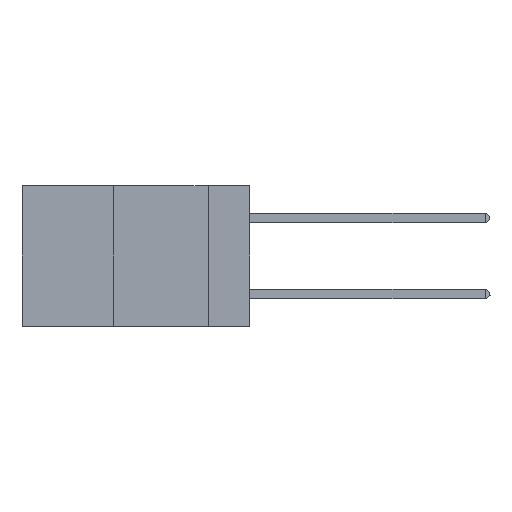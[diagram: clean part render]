
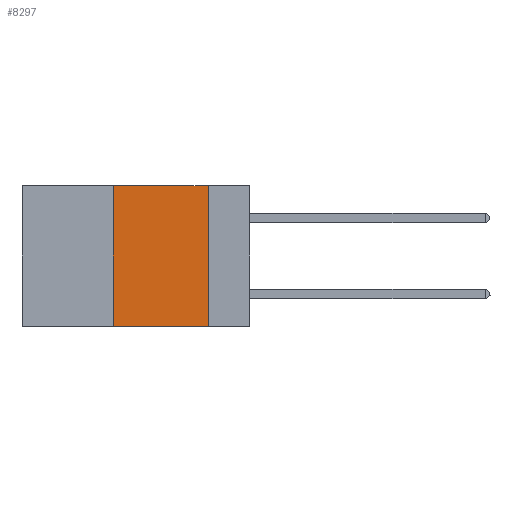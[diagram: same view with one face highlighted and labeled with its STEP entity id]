
A CAD part, left-side view. The second image highlights one B-rep face of the part: STEP entity #8297.
In plain terms, the highlighted planar face has unit normal (-1, 0, 0).
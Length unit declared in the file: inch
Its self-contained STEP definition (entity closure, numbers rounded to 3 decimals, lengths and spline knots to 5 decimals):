
#492 = DIRECTION ( 'NONE',  ( 0., 0., 1. ) ) ;
#702 = VECTOR ( 'NONE', #6221, 39.37008 ) ;
#776 = ORIENTED_EDGE ( 'NONE', *, *, #14512, .F. ) ;
#954 = EDGE_LOOP ( 'NONE', ( #1184, #1375, #776, #11530 ) ) ;
#1025 = CARTESIAN_POINT ( 'NONE',  ( 0., 0.11, 0. ) ) ;
#1184 = ORIENTED_EDGE ( 'NONE', *, *, #7351, .F. ) ;
#1375 = ORIENTED_EDGE ( 'NONE', *, *, #3926, .F. ) ;
#1464 = CARTESIAN_POINT ( 'NONE',  ( 0., 0.11, -0.37 ) ) ;
#1630 = CARTESIAN_POINT ( 'NONE',  ( 0., 0.36, 0. ) ) ;
#2673 = VECTOR ( 'NONE', #4541, 39.37008 ) ;
#2970 = VERTEX_POINT ( 'NONE', #3033 ) ;
#3033 = CARTESIAN_POINT ( 'NONE',  ( 0., 0.36, -0.37 ) ) ;
#3047 = CARTESIAN_POINT ( 'NONE',  ( 0., 0.6, 0. ) ) ;
#3343 = CARTESIAN_POINT ( 'NONE',  ( 0., 0.11, 0. ) ) ;
#3744 = VERTEX_POINT ( 'NONE', #1464 ) ;
#3909 = CARTESIAN_POINT ( 'NONE',  ( 0., 0.6, -0.37 ) ) ;
#3926 = EDGE_CURVE ( 'NONE', #8511, #8429, #7012, .T. ) ;
#4541 = DIRECTION ( 'NONE',  ( 0., 0., -1. ) ) ;
#6221 = DIRECTION ( 'NONE',  ( 0., -1., 0. ) ) ;
#6929 = CARTESIAN_POINT ( 'NONE',  ( 0., 0.36, 0. ) ) ;
#7012 = LINE ( 'NONE', #15236, #8849 ) ;
#7351 = EDGE_CURVE ( 'NONE', #8429, #3744, #13919, .T. ) ;
#7542 = LINE ( 'NONE', #1630, #14424 ) ;
#8297 = ADVANCED_FACE ( 'NONE', ( #9582 ), #10255, .F. ) ;
#8429 = VERTEX_POINT ( 'NONE', #1025 ) ;
#8511 = VERTEX_POINT ( 'NONE', #6929 ) ;
#8849 = VECTOR ( 'NONE', #14131, 39.37008 ) ;
#9582 = FACE_OUTER_BOUND ( 'NONE', #954, .T. ) ;
#9937 = LINE ( 'NONE', #3909, #702 ) ;
#10255 = PLANE ( 'NONE',  #12591 ) ;
#11530 = ORIENTED_EDGE ( 'NONE', *, *, #14895, .T. ) ;
#12591 = AXIS2_PLACEMENT_3D ( 'NONE', #3047, #13897, #15010 ) ;
#13897 = DIRECTION ( 'NONE',  ( 1., 0., 0. ) ) ;
#13919 = LINE ( 'NONE', #3343, #2673 ) ;
#14131 = DIRECTION ( 'NONE',  ( 0., -1., 0. ) ) ;
#14424 = VECTOR ( 'NONE', #492, 39.37008 ) ;
#14512 = EDGE_CURVE ( 'NONE', #2970, #8511, #7542, .T. ) ;
#14895 = EDGE_CURVE ( 'NONE', #2970, #3744, #9937, .T. ) ;
#15010 = DIRECTION ( 'NONE',  ( 0., 0., -1. ) ) ;
#15236 = CARTESIAN_POINT ( 'NONE',  ( 0., 0.6, 0. ) ) ;
